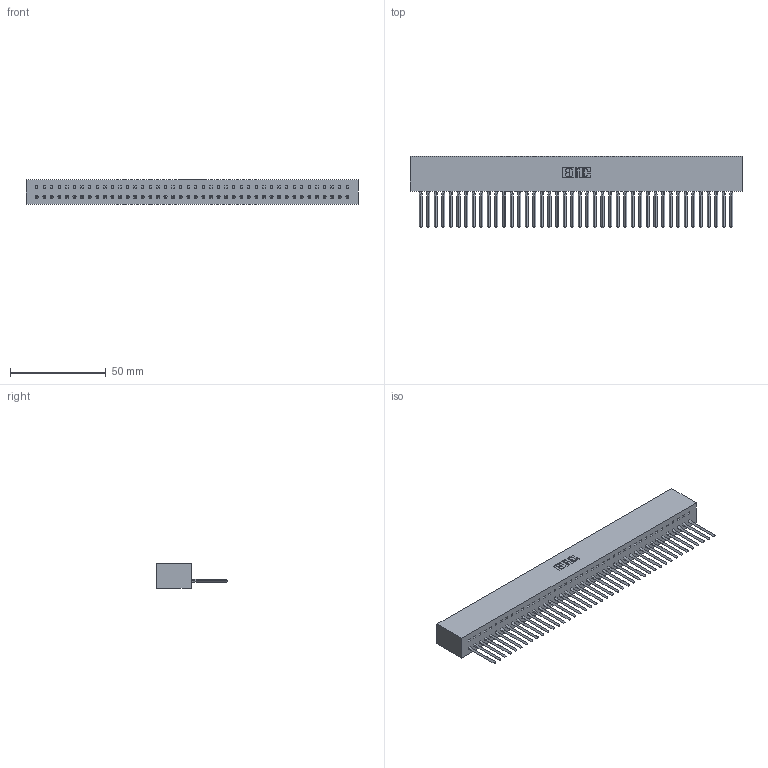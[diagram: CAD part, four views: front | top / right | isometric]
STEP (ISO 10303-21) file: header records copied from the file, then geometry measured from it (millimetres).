
FILE_DESCRIPTION (( 'STEP AP203' ), '1' );
FILE_NAME ('317-042-541-601.STEP', '2020-02-28T01:10:07', ( '' ), ( '' ), 'SwSTEP 2.0', 'SolidWorks 2016', '' );
FILE_SCHEMA (( 'CONFIG_CONTROL_DESIGN' ));
Products named in the file (3): 317-290-002_541; 317 Part_Lugless; 317-042-541-601
Assembly tree (43 placements, depth 2):
  317-042-541-601
    317 Part_Lugless
    317-290-002_541  x42
Bounding box: 173.63 x 37.34 x 12.7 mm (x, y, z)
Volume: 29863.5 mm3; surface area: 42392.8 mm2
Topology: 43 solids, 43 shells, 6474 faces, 18467 edges, 12002 vertices
Faces by surface type: plane 5258, cylinder 1048, bspline 168
Entity records: 60506 total; most frequent: CARTESIAN_POINT 11399, ORIENTED_EDGE 10694, DIRECTION 8775, EDGE_CURVE 5347, VECTOR 4991, LINE 4991, VERTEX_POINT 3556, AXIS2_PLACEMENT_3D 1892
